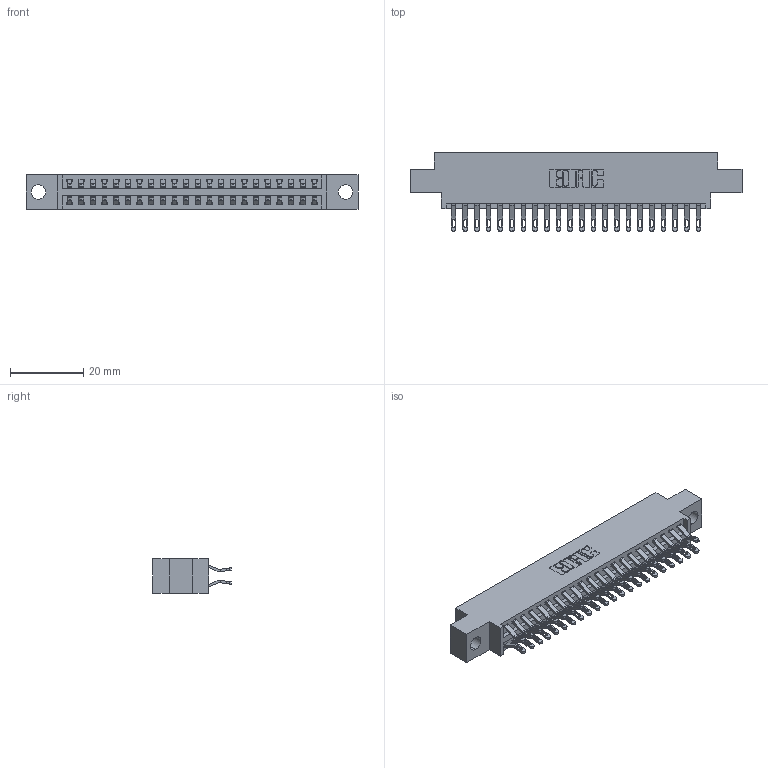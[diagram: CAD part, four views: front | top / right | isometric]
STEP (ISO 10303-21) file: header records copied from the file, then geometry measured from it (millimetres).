
FILE_DESCRIPTION (( 'STEP AP203' ), '1' );
FILE_NAME ('396-044-555-804.STEP', '2018-09-07T04:49:41', ( '' ), ( '' ), 'SwSTEP 2.0', 'SolidWorks 2016', '' );
FILE_SCHEMA (( 'CONFIG_CONTROL_DESIGN' ));
Length unit declared in the file: inch
Products named in the file (3): 346 Part_0.170 Offset - 0.156 Dia-TH; 345-292-001_555 Tail; 396-044-555-804
Assembly tree (45 placements, depth 2):
  396-044-555-804
    346 Part_0.170 Offset - 0.156 Dia-TH
    345-292-001_555 Tail  x44
Bounding box: 90.42 x 21.46 x 9.4 mm (x, y, z)
Volume: 8547.3 mm3; surface area: 11882.4 mm2
Topology: 45 solids, 45 shells, 2678 faces, 8393 edges, 5594 vertices
Faces by surface type: plane 1532, cylinder 1146
Entity records: 17511 total; most frequent: CARTESIAN_POINT 2950, ORIENTED_EDGE 2854, DIRECTION 2619, EDGE_CURVE 1427, VECTOR 1187, LINE 1187, VERTEX_POINT 950, AXIS2_PLACEMENT_3D 716
